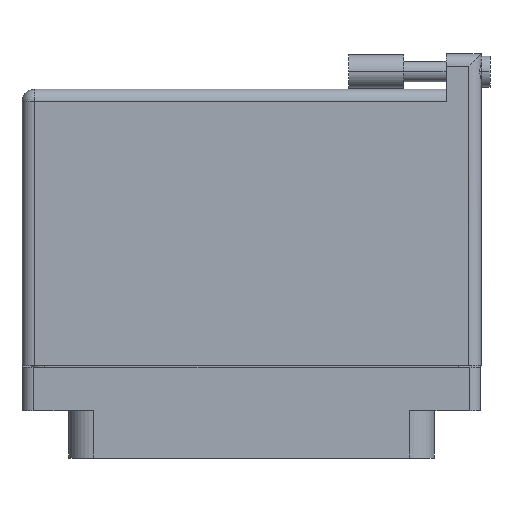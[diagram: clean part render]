
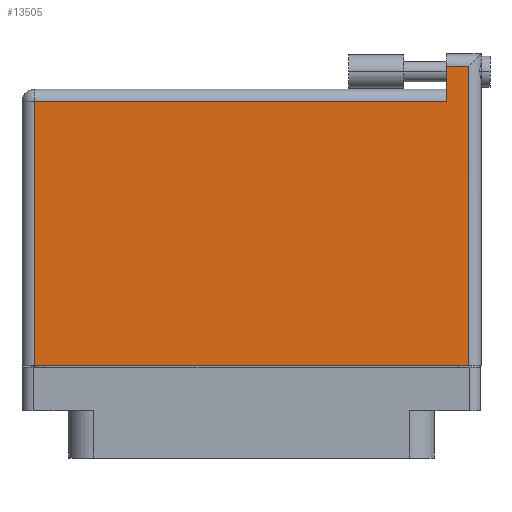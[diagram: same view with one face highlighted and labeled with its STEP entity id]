
A CAD part, front view. The second image highlights one B-rep face of the part: STEP entity #13505.
In plain terms, the highlighted face is planar.
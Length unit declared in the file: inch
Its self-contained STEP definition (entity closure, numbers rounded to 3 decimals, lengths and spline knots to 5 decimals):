
#3690 = ORIENTED_EDGE ( 'NONE', *, *, #22568, .T. ) ;
#4485 = ORIENTED_EDGE ( 'NONE', *, *, #26246, .T. ) ;
#4752 = FACE_OUTER_BOUND ( 'NONE', #10934, .T. ) ;
#5912 = LINE ( 'NONE', #28533, #33425 ) ;
#6949 = EDGE_CURVE ( 'NONE', #27198, #24694, #35426, .T. ) ;
#7481 = DIRECTION ( 'NONE',  ( -1., 0., 0. ) ) ;
#7862 = VERTEX_POINT ( 'NONE', #44165 ) ;
#9336 = CARTESIAN_POINT ( 'NONE',  ( 1.103, 1.666, 0.4495 ) ) ;
#9451 = VECTOR ( 'NONE', #7481, 39.37008 ) ;
#10934 = EDGE_LOOP ( 'NONE', ( #43578, #42322, #4485, #12376, #3690, #26551 ) ) ;
#12020 = CARTESIAN_POINT ( 'NONE',  ( -1.3, 1.596, 0.4495 ) ) ;
#12376 = ORIENTED_EDGE ( 'NONE', *, *, #6949, .T. ) ;
#12462 = DIRECTION ( 'NONE',  ( 0., -1., 0. ) ) ;
#12837 = CARTESIAN_POINT ( 'NONE',  ( 1.23, 1.596, 0.4495 ) ) ;
#13505 = ADVANCED_FACE ( 'NONE', ( #4752 ), #51504, .F. ) ;
#14403 = LINE ( 'NONE', #12020, #9451 ) ;
#18219 = CARTESIAN_POINT ( 'NONE',  ( -1.3, -0.1, 0.4495 ) ) ;
#18408 = CARTESIAN_POINT ( 'NONE',  ( -1.23, 1.396, 0.4495 ) ) ;
#20176 = EDGE_CURVE ( 'NONE', #7862, #43722, #24635, .T. ) ;
#22568 = EDGE_CURVE ( 'NONE', #24694, #33195, #34281, .T. ) ;
#24423 = AXIS2_PLACEMENT_3D ( 'NONE', #39945, #31642, #44041 ) ;
#24635 = LINE ( 'NONE', #18219, #39088 ) ;
#24694 = VERTEX_POINT ( 'NONE', #36032 ) ;
#24789 = VECTOR ( 'NONE', #12462, 39.37008 ) ;
#26246 = EDGE_CURVE ( 'NONE', #41142, #27198, #14403, .T. ) ;
#26551 = ORIENTED_EDGE ( 'NONE', *, *, #32693, .T. ) ;
#26980 = CARTESIAN_POINT ( 'NONE',  ( 1.23, -0.1, 0.4495 ) ) ;
#27198 = VERTEX_POINT ( 'NONE', #34263 ) ;
#27950 = VECTOR ( 'NONE', #43944, 39.37008 ) ;
#28533 = CARTESIAN_POINT ( 'NONE',  ( 1.23, 1.666, 0.4495 ) ) ;
#28762 = CARTESIAN_POINT ( 'NONE',  ( -1.23, -0.1, 0.4495 ) ) ;
#30478 = DIRECTION ( 'NONE',  ( 1., 0., 0. ) ) ;
#31642 = DIRECTION ( 'NONE',  ( 0., 0., -1. ) ) ;
#32693 = EDGE_CURVE ( 'NONE', #33195, #7862, #32905, .T. ) ;
#32905 = LINE ( 'NONE', #28762, #41660 ) ;
#33195 = VERTEX_POINT ( 'NONE', #18408 ) ;
#33425 = VECTOR ( 'NONE', #35036, 39.37008 ) ;
#34263 = CARTESIAN_POINT ( 'NONE',  ( 1.103, 1.596, 0.4495 ) ) ;
#34281 = LINE ( 'NONE', #40515, #27950 ) ;
#35036 = DIRECTION ( 'NONE',  ( 0., 1., 0. ) ) ;
#35426 = LINE ( 'NONE', #9336, #24789 ) ;
#36032 = CARTESIAN_POINT ( 'NONE',  ( 1.103, 1.396, 0.4495 ) ) ;
#36525 = DIRECTION ( 'NONE',  ( 0., -1., 0. ) ) ;
#38441 = EDGE_CURVE ( 'NONE', #43722, #41142, #5912, .T. ) ;
#39088 = VECTOR ( 'NONE', #30478, 39.37008 ) ;
#39945 = CARTESIAN_POINT ( 'NONE',  ( -1.3, 1.466, 0.4495 ) ) ;
#40515 = CARTESIAN_POINT ( 'NONE',  ( -1.3, 1.396, 0.4495 ) ) ;
#41142 = VERTEX_POINT ( 'NONE', #12837 ) ;
#41660 = VECTOR ( 'NONE', #36525, 39.37008 ) ;
#42322 = ORIENTED_EDGE ( 'NONE', *, *, #38441, .T. ) ;
#43578 = ORIENTED_EDGE ( 'NONE', *, *, #20176, .T. ) ;
#43722 = VERTEX_POINT ( 'NONE', #26980 ) ;
#43944 = DIRECTION ( 'NONE',  ( -1., 0., 0. ) ) ;
#44041 = DIRECTION ( 'NONE',  ( -1., 0., 0. ) ) ;
#44165 = CARTESIAN_POINT ( 'NONE',  ( -1.23, -0.1, 0.4495 ) ) ;
#51504 = PLANE ( 'NONE',  #24423 ) ;
